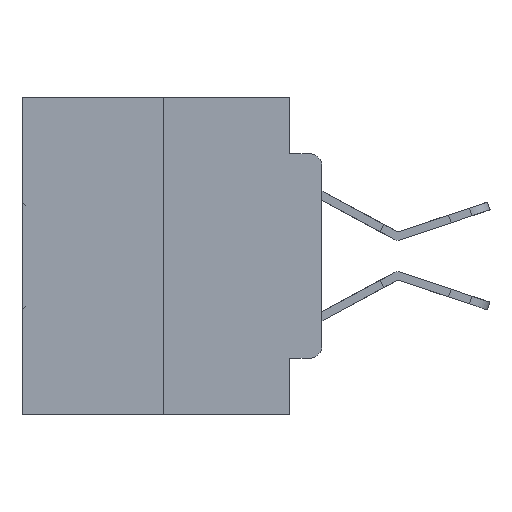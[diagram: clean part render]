
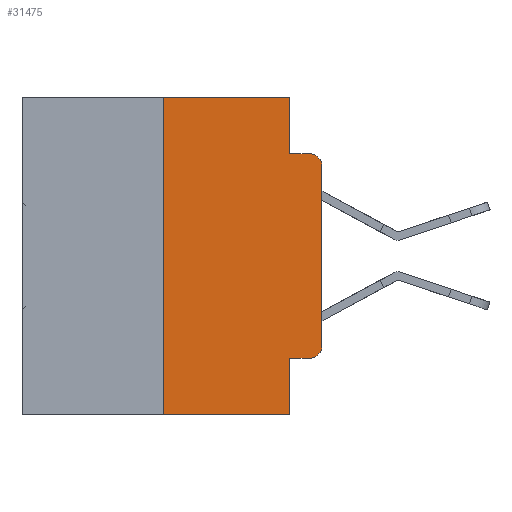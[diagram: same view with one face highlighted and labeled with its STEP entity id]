
A CAD part, left-side view. The second image highlights one B-rep face of the part: STEP entity #31475.
In plain terms, the highlighted planar face has unit normal (-1, 0, 0).
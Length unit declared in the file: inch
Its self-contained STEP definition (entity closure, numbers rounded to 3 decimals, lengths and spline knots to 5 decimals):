
#398 = CARTESIAN_POINT ( 'NONE',  ( 0., 0., 0. ) ) ;
#813 = DIRECTION ( 'NONE',  ( 0., 0., -1. ) ) ;
#841 = CARTESIAN_POINT ( 'NONE',  ( 0., 0.051, 0. ) ) ;
#1336 = EDGE_CURVE ( 'NONE', #10274, #9241, #6692, .T. ) ;
#2196 = DIRECTION ( 'NONE',  ( 1., 0., 0. ) ) ;
#2419 = EDGE_CURVE ( 'NONE', #23636, #9241, #2674, .T. ) ;
#2616 = VECTOR ( 'NONE', #26806, 39.37008 ) ;
#2674 = CIRCLE ( 'NONE', #16361, 0.02 ) ;
#2872 = LINE ( 'NONE', #398, #27786 ) ;
#2954 = LINE ( 'NONE', #12982, #31940 ) ;
#3260 = DIRECTION ( 'NONE',  ( -1., 0., 0. ) ) ;
#3343 = CARTESIAN_POINT ( 'NONE',  ( 0., 0.25, 0. ) ) ;
#3475 = DIRECTION ( 'NONE',  ( 0., 0., -1. ) ) ;
#4054 = CARTESIAN_POINT ( 'NONE',  ( 0., 0.051, -0.0885 ) ) ;
#4655 = CARTESIAN_POINT ( 'NONE',  ( 0., 0.051, -0.5 ) ) ;
#5013 = DIRECTION ( 'NONE',  ( 0., 0., 1. ) ) ;
#5337 = DIRECTION ( 'NONE',  ( 0., -1., 0. ) ) ;
#5607 = CARTESIAN_POINT ( 'NONE',  ( 0., 0.25, -0.5 ) ) ;
#5948 = LINE ( 'NONE', #841, #12397 ) ;
#6080 = ORIENTED_EDGE ( 'NONE', *, *, #18082, .T. ) ;
#6692 = LINE ( 'NONE', #4054, #28576 ) ;
#6777 = DIRECTION ( 'NONE',  ( 0., 0., -1. ) ) ;
#6999 = EDGE_CURVE ( 'NONE', #27260, #18355, #5948, .T. ) ;
#7018 = VERTEX_POINT ( 'NONE', #5607 ) ;
#7734 = EDGE_LOOP ( 'NONE', ( #6080, #26891, #20292, #20396, #28371, #26706, #12664, #14345, #13331, #31227 ) ) ;
#9241 = VERTEX_POINT ( 'NONE', #12051 ) ;
#9963 = LINE ( 'NONE', #20173, #22527 ) ;
#10245 = EDGE_CURVE ( 'NONE', #27260, #19130, #30712, .T. ) ;
#10274 = VERTEX_POINT ( 'NONE', #17683 ) ;
#10426 = DIRECTION ( 'NONE',  ( 0., 0., 1. ) ) ;
#11491 = CARTESIAN_POINT ( 'NONE',  ( 0., 0.02, -0.4115 ) ) ;
#12051 = CARTESIAN_POINT ( 'NONE',  ( 0., 0.02, -0.0885 ) ) ;
#12397 = VECTOR ( 'NONE', #3475, 39.37008 ) ;
#12405 = CARTESIAN_POINT ( 'NONE',  ( 0., 0.051, -0.4115 ) ) ;
#12516 = CARTESIAN_POINT ( 'NONE',  ( 0., 0.473, 0. ) ) ;
#12664 = ORIENTED_EDGE ( 'NONE', *, *, #15627, .T. ) ;
#12982 = CARTESIAN_POINT ( 'NONE',  ( 0., 0.051, 0. ) ) ;
#13284 = DIRECTION ( 'NONE',  ( 0., 0., -1. ) ) ;
#13331 = ORIENTED_EDGE ( 'NONE', *, *, #10245, .T. ) ;
#14228 = EDGE_CURVE ( 'NONE', #19130, #29391, #29405, .T. ) ;
#14345 = ORIENTED_EDGE ( 'NONE', *, *, #6999, .F. ) ;
#14865 = EDGE_CURVE ( 'NONE', #25537, #19280, #22909, .T. ) ;
#14936 = CARTESIAN_POINT ( 'NONE',  ( 0., 0.051, 0. ) ) ;
#15627 = EDGE_CURVE ( 'NONE', #7018, #18355, #19862, .T. ) ;
#16361 = AXIS2_PLACEMENT_3D ( 'NONE', #32334, #32006, #6777 ) ;
#17040 = CARTESIAN_POINT ( 'NONE',  ( 0., 0.051, -0.4115 ) ) ;
#17493 = DIRECTION ( 'NONE',  ( 0., 0., -1. ) ) ;
#17683 = CARTESIAN_POINT ( 'NONE',  ( 0., 0.051, -0.0885 ) ) ;
#18082 = EDGE_CURVE ( 'NONE', #29391, #23636, #2872, .T. ) ;
#18355 = VERTEX_POINT ( 'NONE', #4655 ) ;
#19130 = VERTEX_POINT ( 'NONE', #11491 ) ;
#19280 = VERTEX_POINT ( 'NONE', #14936 ) ;
#19434 = VECTOR ( 'NONE', #30493, 39.37008 ) ;
#19862 = LINE ( 'NONE', #26639, #2616 ) ;
#20016 = CARTESIAN_POINT ( 'NONE',  ( 0., 0., -0.1085 ) ) ;
#20173 = CARTESIAN_POINT ( 'NONE',  ( 0., 0.25, 0. ) ) ;
#20292 = ORIENTED_EDGE ( 'NONE', *, *, #1336, .F. ) ;
#20396 = ORIENTED_EDGE ( 'NONE', *, *, #22838, .F. ) ;
#20746 = CARTESIAN_POINT ( 'NONE',  ( 0., 0.473, 0. ) ) ;
#21070 = AXIS2_PLACEMENT_3D ( 'NONE', #12516, #2196, #17493 ) ;
#22527 = VECTOR ( 'NONE', #5013, 39.37008 ) ;
#22838 = EDGE_CURVE ( 'NONE', #19280, #10274, #2954, .T. ) ;
#22909 = LINE ( 'NONE', #20746, #19434 ) ;
#23568 = EDGE_CURVE ( 'NONE', #7018, #25537, #9963, .T. ) ;
#23572 = CARTESIAN_POINT ( 'NONE',  ( 0., 0., -0.3915 ) ) ;
#23636 = VERTEX_POINT ( 'NONE', #20016 ) ;
#25537 = VERTEX_POINT ( 'NONE', #3343 ) ;
#26639 = CARTESIAN_POINT ( 'NONE',  ( 0., 0.473, -0.5 ) ) ;
#26706 = ORIENTED_EDGE ( 'NONE', *, *, #23568, .F. ) ;
#26806 = DIRECTION ( 'NONE',  ( 0., -1., 0. ) ) ;
#26891 = ORIENTED_EDGE ( 'NONE', *, *, #2419, .T. ) ;
#27064 = PLANE ( 'NONE',  #21070 ) ;
#27260 = VERTEX_POINT ( 'NONE', #17040 ) ;
#27390 = FACE_OUTER_BOUND ( 'NONE', #7734, .T. ) ;
#27786 = VECTOR ( 'NONE', #10426, 39.37008 ) ;
#28371 = ORIENTED_EDGE ( 'NONE', *, *, #14865, .F. ) ;
#28576 = VECTOR ( 'NONE', #28802, 39.37008 ) ;
#28796 = CARTESIAN_POINT ( 'NONE',  ( 0., 0.02, -0.3915 ) ) ;
#28802 = DIRECTION ( 'NONE',  ( 0., -1., 0. ) ) ;
#29391 = VERTEX_POINT ( 'NONE', #23572 ) ;
#29405 = CIRCLE ( 'NONE', #30428, 0.02 ) ;
#30428 = AXIS2_PLACEMENT_3D ( 'NONE', #28796, #3260, #13284 ) ;
#30493 = DIRECTION ( 'NONE',  ( 0., -1., 0. ) ) ;
#30712 = LINE ( 'NONE', #12405, #31138 ) ;
#31138 = VECTOR ( 'NONE', #5337, 39.37008 ) ;
#31227 = ORIENTED_EDGE ( 'NONE', *, *, #14228, .T. ) ;
#31475 = ADVANCED_FACE ( 'NONE', ( #27390 ), #27064, .F. ) ;
#31940 = VECTOR ( 'NONE', #813, 39.37008 ) ;
#32006 = DIRECTION ( 'NONE',  ( -1., 0., 0. ) ) ;
#32334 = CARTESIAN_POINT ( 'NONE',  ( 0., 0.02, -0.1085 ) ) ;
